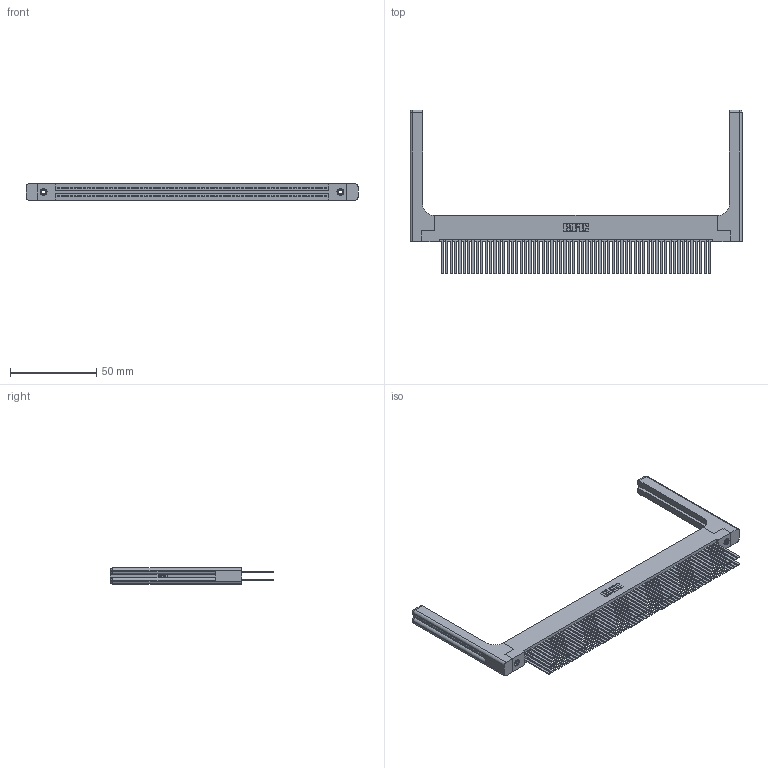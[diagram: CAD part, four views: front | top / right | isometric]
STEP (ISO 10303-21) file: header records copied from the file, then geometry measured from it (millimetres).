
FILE_DESCRIPTION (( 'STEP AP203' ), '1' );
FILE_NAME ('395-124-544-258.STEP', '2019-10-28T12:07:15', ( '' ), ( '' ), 'SwSTEP 2.0', 'SolidWorks 2016', '' );
FILE_SCHEMA (( 'CONFIG_CONTROL_DESIGN' ));
Length unit declared in the file: inch
Products named in the file (5): 345-250-001_345-250-001-102; 345-220-058_345-220-058; 395-124-544-258; 345 Part_Flush Mounting Lugs - 0.156 Dia-TH; 345-292-001_345-293-144
Assembly tree (129 placements, depth 2):
  395-124-544-258
    345 Part_Flush Mounting Lugs - 0.156 Dia-TH
    345-292-001_345-293-144  x124
    345-250-001_345-250-001-102  x2
    345-220-058_345-220-058  x2
Bounding box: 192.51 x 94.92 x 9.4 mm (x, y, z)
Volume: 29099.3 mm3; surface area: 41026.9 mm2
Topology: 129 solids, 129 shells, 5838 faces, 17251 edges, 11314 vertices
Faces by surface type: plane 3824, cylinder 1954, bspline 36, cone 12, sphere 8, torus 4
Entity records: 50952 total; most frequent: CARTESIAN_POINT 9513, ORIENTED_EDGE 8244, DIRECTION 7294, EDGE_CURVE 4122, LINE 3654, VECTOR 3654, VERTEX_POINT 2738, AXIS2_PLACEMENT_3D 1820
